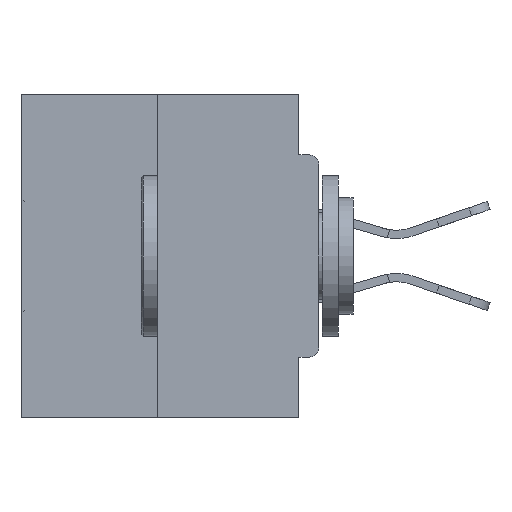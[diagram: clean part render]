
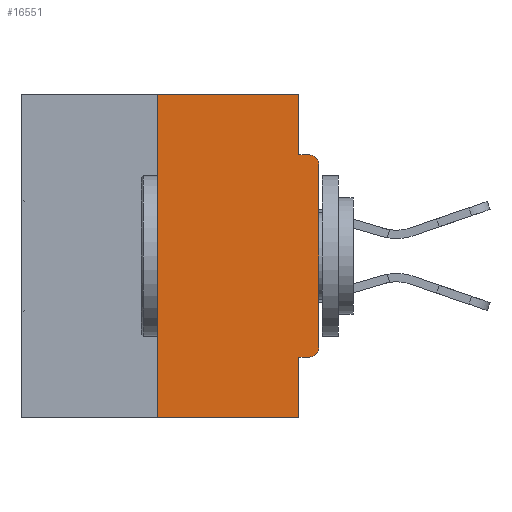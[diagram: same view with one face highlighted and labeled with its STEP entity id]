
A CAD part, left-side view. The second image highlights one B-rep face of the part: STEP entity #16551.
In plain terms, the highlighted planar face has unit normal (-1, 0, 0).
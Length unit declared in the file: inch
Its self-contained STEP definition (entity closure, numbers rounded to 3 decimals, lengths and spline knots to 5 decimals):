
#87 = DIRECTION ( 'NONE',  ( -1., 0., 0. ) ) ;
#165 = VECTOR ( 'NONE', #24212, 39.37008 ) ;
#216 = EDGE_CURVE ( 'NONE', #37863, #19433, #34239, .T. ) ;
#740 = DIRECTION ( 'NONE',  ( 0., 0., -1. ) ) ;
#892 = ORIENTED_EDGE ( 'NONE', *, *, #3987, .T. ) ;
#1363 = LINE ( 'NONE', #4126, #3416 ) ;
#3401 = DIRECTION ( 'NONE',  ( 0., 0., 1. ) ) ;
#3416 = VECTOR ( 'NONE', #7284, 39.37008 ) ;
#3578 = CARTESIAN_POINT ( 'NONE',  ( 0., 0.015, -0.4065 ) ) ;
#3704 = CARTESIAN_POINT ( 'NONE',  ( 0., 0.015, -0.3915 ) ) ;
#3752 = ORIENTED_EDGE ( 'NONE', *, *, #6321, .F. ) ;
#3898 = CARTESIAN_POINT ( 'NONE',  ( 0., 0.031, 0. ) ) ;
#3987 = EDGE_CURVE ( 'NONE', #12505, #10314, #8395, .T. ) ;
#4126 = CARTESIAN_POINT ( 'NONE',  ( 0., 0.031, -0.5 ) ) ;
#4352 = CARTESIAN_POINT ( 'NONE',  ( 0., 0.031, -0.0935 ) ) ;
#4860 = LINE ( 'NONE', #7208, #32499 ) ;
#5945 = EDGE_CURVE ( 'NONE', #30229, #23847, #4860, .T. ) ;
#6321 = EDGE_CURVE ( 'NONE', #33819, #14821, #15506, .T. ) ;
#7208 = CARTESIAN_POINT ( 'NONE',  ( 0., 0., -0.0935 ) ) ;
#7284 = DIRECTION ( 'NONE',  ( 0., 0., -1. ) ) ;
#7316 = DIRECTION ( 'NONE',  ( 1., 0., 0. ) ) ;
#8047 = EDGE_CURVE ( 'NONE', #10314, #23847, #19426, .T. ) ;
#8395 = LINE ( 'NONE', #14918, #12428 ) ;
#8748 = CARTESIAN_POINT ( 'NONE',  ( 0., 0.46, -0.5 ) ) ;
#9850 = CARTESIAN_POINT ( 'NONE',  ( 0., 0.25, 0. ) ) ;
#10233 = EDGE_CURVE ( 'NONE', #37863, #12505, #34690, .T. ) ;
#10272 = EDGE_CURVE ( 'NONE', #19433, #31804, #1363, .T. ) ;
#10314 = VERTEX_POINT ( 'NONE', #36470 ) ;
#10322 = PLANE ( 'NONE',  #37969 ) ;
#11531 = DIRECTION ( 'NONE',  ( 0., 1., 0. ) ) ;
#12165 = EDGE_CURVE ( 'NONE', #14821, #27709, #35042, .T. ) ;
#12428 = VECTOR ( 'NONE', #27871, 39.37008 ) ;
#12505 = VERTEX_POINT ( 'NONE', #32358 ) ;
#13366 = EDGE_LOOP ( 'NONE', ( #34283, #3752, #25446, #25127, #28949, #40740, #892, #42209, #38736, #23372 ) ) ;
#14821 = VERTEX_POINT ( 'NONE', #17133 ) ;
#14859 = CARTESIAN_POINT ( 'NONE',  ( 0., 0.46, 0. ) ) ;
#14918 = CARTESIAN_POINT ( 'NONE',  ( 0., 0., 0. ) ) ;
#15124 = EDGE_CURVE ( 'NONE', #33819, #31804, #24523, .T. ) ;
#15506 = LINE ( 'NONE', #9850, #27381 ) ;
#16551 = ADVANCED_FACE ( 'NONE', ( #28547 ), #10322, .F. ) ;
#16703 = DIRECTION ( 'NONE',  ( 0., 0., -1. ) ) ;
#17133 = CARTESIAN_POINT ( 'NONE',  ( 0., 0.25, 0. ) ) ;
#17239 = CARTESIAN_POINT ( 'NONE',  ( 0., 0.015, -0.1085 ) ) ;
#18269 = CARTESIAN_POINT ( 'NONE',  ( 0., 0.25, -0.5 ) ) ;
#19426 = CIRCLE ( 'NONE', #42013, 0.015 ) ;
#19433 = VERTEX_POINT ( 'NONE', #23243 ) ;
#20130 = DIRECTION ( 'NONE',  ( 0., 0., -1. ) ) ;
#20203 = DIRECTION ( 'NONE',  ( 0., -1., 0. ) ) ;
#21236 = CARTESIAN_POINT ( 'NONE',  ( 0., 0., -0.4065 ) ) ;
#22170 = DIRECTION ( 'NONE',  ( 0., -1., 0. ) ) ;
#23243 = CARTESIAN_POINT ( 'NONE',  ( 0., 0.031, -0.4065 ) ) ;
#23372 = ORIENTED_EDGE ( 'NONE', *, *, #39206, .F. ) ;
#23847 = VERTEX_POINT ( 'NONE', #35349 ) ;
#23934 = VECTOR ( 'NONE', #740, 39.37008 ) ;
#24212 = DIRECTION ( 'NONE',  ( 0., -1., 0. ) ) ;
#24523 = LINE ( 'NONE', #8748, #32222 ) ;
#25127 = ORIENTED_EDGE ( 'NONE', *, *, #10272, .F. ) ;
#25446 = ORIENTED_EDGE ( 'NONE', *, *, #15124, .T. ) ;
#27381 = VECTOR ( 'NONE', #3401, 39.37008 ) ;
#27709 = VERTEX_POINT ( 'NONE', #29063 ) ;
#27871 = DIRECTION ( 'NONE',  ( 0., 0., 1. ) ) ;
#28547 = FACE_OUTER_BOUND ( 'NONE', #13366, .T. ) ;
#28949 = ORIENTED_EDGE ( 'NONE', *, *, #216, .F. ) ;
#29063 = CARTESIAN_POINT ( 'NONE',  ( 0., 0.031, 0. ) ) ;
#29473 = DIRECTION ( 'NONE',  ( 0., 0., -1. ) ) ;
#30210 = DIRECTION ( 'NONE',  ( -1., 0., 0. ) ) ;
#30229 = VERTEX_POINT ( 'NONE', #4352 ) ;
#31804 = VERTEX_POINT ( 'NONE', #40081 ) ;
#32222 = VECTOR ( 'NONE', #22170, 39.37008 ) ;
#32358 = CARTESIAN_POINT ( 'NONE',  ( 0., 0., -0.3915 ) ) ;
#32499 = VECTOR ( 'NONE', #20203, 39.37008 ) ;
#32948 = CARTESIAN_POINT ( 'NONE',  ( 0., 0.46, 0. ) ) ;
#33194 = VECTOR ( 'NONE', #11531, 39.37008 ) ;
#33674 = LINE ( 'NONE', #3898, #23934 ) ;
#33819 = VERTEX_POINT ( 'NONE', #18269 ) ;
#34239 = LINE ( 'NONE', #21236, #33194 ) ;
#34283 = ORIENTED_EDGE ( 'NONE', *, *, #12165, .F. ) ;
#34690 = CIRCLE ( 'NONE', #39921, 0.015 ) ;
#35042 = LINE ( 'NONE', #14859, #165 ) ;
#35349 = CARTESIAN_POINT ( 'NONE',  ( 0., 0.015, -0.0935 ) ) ;
#36470 = CARTESIAN_POINT ( 'NONE',  ( 0., 0., -0.1085 ) ) ;
#37863 = VERTEX_POINT ( 'NONE', #3578 ) ;
#37969 = AXIS2_PLACEMENT_3D ( 'NONE', #32948, #7316, #16703 ) ;
#38736 = ORIENTED_EDGE ( 'NONE', *, *, #5945, .F. ) ;
#39206 = EDGE_CURVE ( 'NONE', #27709, #30229, #33674, .T. ) ;
#39921 = AXIS2_PLACEMENT_3D ( 'NONE', #3704, #30210, #20130 ) ;
#40081 = CARTESIAN_POINT ( 'NONE',  ( 0., 0.031, -0.5 ) ) ;
#40740 = ORIENTED_EDGE ( 'NONE', *, *, #10233, .T. ) ;
#42013 = AXIS2_PLACEMENT_3D ( 'NONE', #17239, #87, #29473 ) ;
#42209 = ORIENTED_EDGE ( 'NONE', *, *, #8047, .T. ) ;
